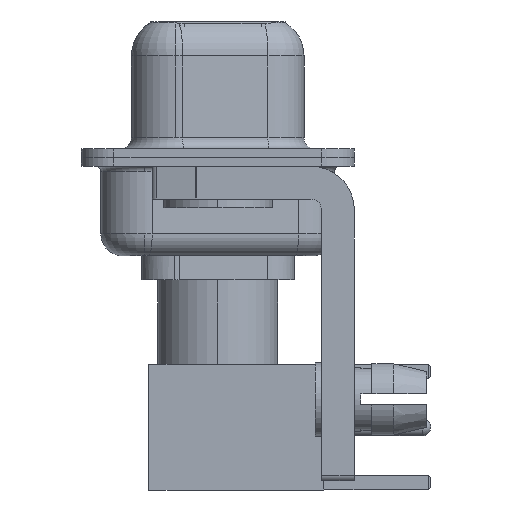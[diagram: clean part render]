
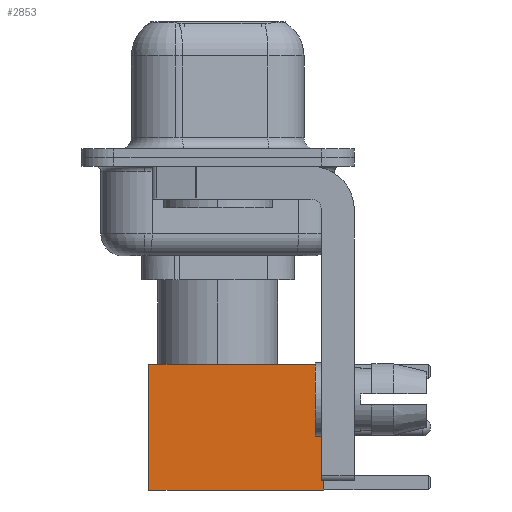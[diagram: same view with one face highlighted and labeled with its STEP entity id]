
A CAD part, left-side view. The second image highlights one B-rep face of the part: STEP entity #2853.
In plain terms, the highlighted face is planar.
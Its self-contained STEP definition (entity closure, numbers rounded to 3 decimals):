
#492 = VECTOR ( 'NONE', #17551, 1000. ) ;
#990 = CARTESIAN_POINT ( 'NONE',  ( 2.875, 2.875, 0. ) ) ;
#1157 = DIRECTION ( 'NONE',  ( 0., 1., 0. ) ) ;
#1577 = CARTESIAN_POINT ( 'NONE',  ( 0., 2.875, 8. ) ) ;
#1821 = PLANE ( 'NONE',  #10234 ) ;
#2281 = LINE ( 'NONE', #990, #492 ) ;
#2591 = ORIENTED_EDGE ( 'NONE', *, *, #12688, .T. ) ;
#2853 = ADVANCED_FACE ( 'NONE', ( #4204 ), #1821, .T. ) ;
#4204 = FACE_OUTER_BOUND ( 'NONE', #16546, .T. ) ;
#4922 = DIRECTION ( 'NONE',  ( 0., 0., -1. ) ) ;
#6290 = VERTEX_POINT ( 'NONE', #18540 ) ;
#6511 = VECTOR ( 'NONE', #14542, 1000. ) ;
#6515 = EDGE_CURVE ( 'NONE', #13519, #11706, #8052, .T. ) ;
#7566 = DIRECTION ( 'NONE',  ( -1., 0., 0. ) ) ;
#8052 = LINE ( 'NONE', #12554, #12730 ) ;
#8202 = EDGE_CURVE ( 'NONE', #13919, #13519, #19215, .T. ) ;
#9023 = CARTESIAN_POINT ( 'NONE',  ( -2.875, 2.875, 0. ) ) ;
#9214 = ORIENTED_EDGE ( 'NONE', *, *, #6515, .F. ) ;
#10234 = AXIS2_PLACEMENT_3D ( 'NONE', #13576, #1157, #16051 ) ;
#10575 = VECTOR ( 'NONE', #7566, 1000. ) ;
#11414 = LINE ( 'NONE', #17385, #6511 ) ;
#11706 = VERTEX_POINT ( 'NONE', #9023 ) ;
#12527 = ORIENTED_EDGE ( 'NONE', *, *, #14588, .T. ) ;
#12554 = CARTESIAN_POINT ( 'NONE',  ( -2.875, 2.875, 0. ) ) ;
#12688 = EDGE_CURVE ( 'NONE', #6290, #11706, #11414, .T. ) ;
#12730 = VECTOR ( 'NONE', #4922, 1000. ) ;
#13519 = VERTEX_POINT ( 'NONE', #14210 ) ;
#13576 = CARTESIAN_POINT ( 'NONE',  ( 2.875, 2.875, 0. ) ) ;
#13919 = VERTEX_POINT ( 'NONE', #16872 ) ;
#14210 = CARTESIAN_POINT ( 'NONE',  ( -2.875, 2.875, 8. ) ) ;
#14542 = DIRECTION ( 'NONE',  ( -1., 0., 0. ) ) ;
#14551 = ORIENTED_EDGE ( 'NONE', *, *, #8202, .F. ) ;
#14588 = EDGE_CURVE ( 'NONE', #13919, #6290, #2281, .T. ) ;
#16051 = DIRECTION ( 'NONE',  ( 0., 0., 1. ) ) ;
#16546 = EDGE_LOOP ( 'NONE', ( #12527, #2591, #9214, #14551 ) ) ;
#16872 = CARTESIAN_POINT ( 'NONE',  ( 2.875, 2.875, 8. ) ) ;
#17385 = CARTESIAN_POINT ( 'NONE',  ( 0., 2.875, 0. ) ) ;
#17551 = DIRECTION ( 'NONE',  ( 0., 0., -1. ) ) ;
#18540 = CARTESIAN_POINT ( 'NONE',  ( 2.875, 2.875, 0. ) ) ;
#19215 = LINE ( 'NONE', #1577, #10575 ) ;
